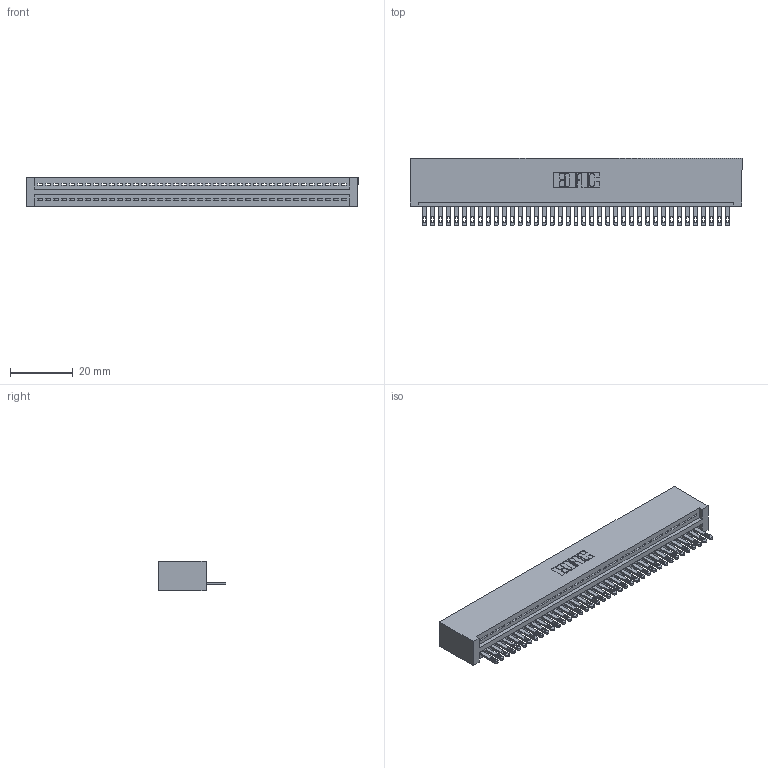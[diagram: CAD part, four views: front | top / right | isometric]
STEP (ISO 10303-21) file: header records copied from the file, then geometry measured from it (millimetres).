
FILE_DESCRIPTION (( 'STEP AP203' ), '1' );
FILE_NAME ('345-039-500-101.STEP', '2019-10-08T05:06:55', ( '' ), ( '' ), 'SwSTEP 2.0', 'SolidWorks 2016', '' );
FILE_SCHEMA (( 'CONFIG_CONTROL_DESIGN' ));
Length unit declared in the file: inch
Products named in the file (3): 345-292-001_345-293-100; 345 Part_No Mounting Lugs; 345-039-500-101
Assembly tree (40 placements, depth 2):
  345-039-500-101
    345 Part_No Mounting Lugs
    345-292-001_345-293-100  x39
Bounding box: 105.66 x 21.51 x 9.4 mm (x, y, z)
Volume: 10620 mm3; surface area: 14350 mm2
Topology: 40 solids, 40 shells, 2224 faces, 6869 edges, 4578 vertices
Faces by surface type: plane 1402, cylinder 822
Entity records: 29409 total; most frequent: CARTESIAN_POINT 5101, ORIENTED_EDGE 5074, DIRECTION 4455, EDGE_CURVE 2537, VECTOR 2253, LINE 2253, VERTEX_POINT 1690, AXIS2_PLACEMENT_3D 1101
